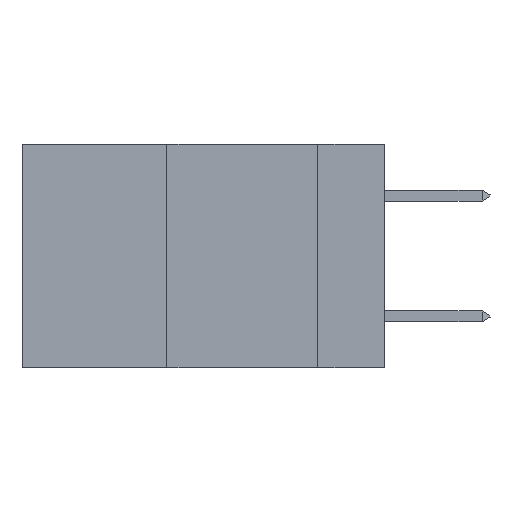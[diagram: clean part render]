
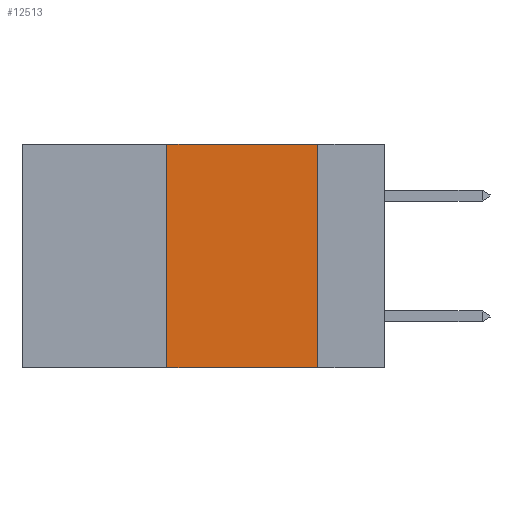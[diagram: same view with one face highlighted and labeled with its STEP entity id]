
A CAD part, left-side view. The second image highlights one B-rep face of the part: STEP entity #12513.
In plain terms, the highlighted planar face has unit normal (-1, 0, 0).
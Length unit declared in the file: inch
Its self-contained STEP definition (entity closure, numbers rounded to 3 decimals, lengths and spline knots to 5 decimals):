
#464 = EDGE_CURVE ( 'NONE', #12204, #27266, #10231, .T. ) ;
#1735 = VECTOR ( 'NONE', #10343, 39.37008 ) ;
#3041 = DIRECTION ( 'NONE',  ( 0., -1., 0. ) ) ;
#7500 = ORIENTED_EDGE ( 'NONE', *, *, #12651, .F. ) ;
#8186 = VECTOR ( 'NONE', #3041, 39.37008 ) ;
#9714 = CARTESIAN_POINT ( 'NONE',  ( 0., 0.6, 0. ) ) ;
#10231 = LINE ( 'NONE', #30888, #22281 ) ;
#10343 = DIRECTION ( 'NONE',  ( 0., 0., -1. ) ) ;
#10851 = CARTESIAN_POINT ( 'NONE',  ( 0., 0.36, 0. ) ) ;
#10962 = VERTEX_POINT ( 'NONE', #27604 ) ;
#12204 = VERTEX_POINT ( 'NONE', #35267 ) ;
#12381 = EDGE_CURVE ( 'NONE', #27266, #10962, #26448, .T. ) ;
#12513 = ADVANCED_FACE ( 'NONE', ( #17651 ), #21956, .F. ) ;
#12651 = EDGE_CURVE ( 'NONE', #10962, #32378, #21337, .T. ) ;
#13428 = VECTOR ( 'NONE', #23872, 39.37008 ) ;
#14500 = CARTESIAN_POINT ( 'NONE',  ( 0., 0.11, -0.37 ) ) ;
#14709 = EDGE_LOOP ( 'NONE', ( #7500, #20167, #26868, #27205 ) ) ;
#17651 = FACE_OUTER_BOUND ( 'NONE', #14709, .T. ) ;
#17937 = CARTESIAN_POINT ( 'NONE',  ( 0., 0.6, 0. ) ) ;
#18446 = DIRECTION ( 'NONE',  ( 1., 0., 0. ) ) ;
#20167 = ORIENTED_EDGE ( 'NONE', *, *, #12381, .F. ) ;
#21337 = LINE ( 'NONE', #25171, #1735 ) ;
#21457 = DIRECTION ( 'NONE',  ( 0., 0., 1. ) ) ;
#21956 = PLANE ( 'NONE',  #26152 ) ;
#22281 = VECTOR ( 'NONE', #21457, 39.37008 ) ;
#23872 = DIRECTION ( 'NONE',  ( 0., -1., 0. ) ) ;
#25171 = CARTESIAN_POINT ( 'NONE',  ( 0., 0.11, 0. ) ) ;
#26152 = AXIS2_PLACEMENT_3D ( 'NONE', #9714, #18446, #30495 ) ;
#26448 = LINE ( 'NONE', #17937, #13428 ) ;
#26868 = ORIENTED_EDGE ( 'NONE', *, *, #464, .F. ) ;
#27202 = CARTESIAN_POINT ( 'NONE',  ( 0., 0.6, -0.37 ) ) ;
#27205 = ORIENTED_EDGE ( 'NONE', *, *, #29893, .T. ) ;
#27266 = VERTEX_POINT ( 'NONE', #10851 ) ;
#27604 = CARTESIAN_POINT ( 'NONE',  ( 0., 0.11, 0. ) ) ;
#29893 = EDGE_CURVE ( 'NONE', #12204, #32378, #33735, .T. ) ;
#30495 = DIRECTION ( 'NONE',  ( 0., 0., -1. ) ) ;
#30888 = CARTESIAN_POINT ( 'NONE',  ( 0., 0.36, 0. ) ) ;
#32378 = VERTEX_POINT ( 'NONE', #14500 ) ;
#33735 = LINE ( 'NONE', #27202, #8186 ) ;
#35267 = CARTESIAN_POINT ( 'NONE',  ( 0., 0.36, -0.37 ) ) ;
